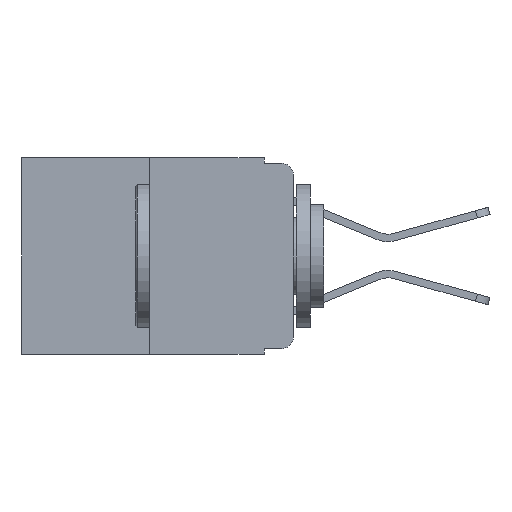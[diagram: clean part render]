
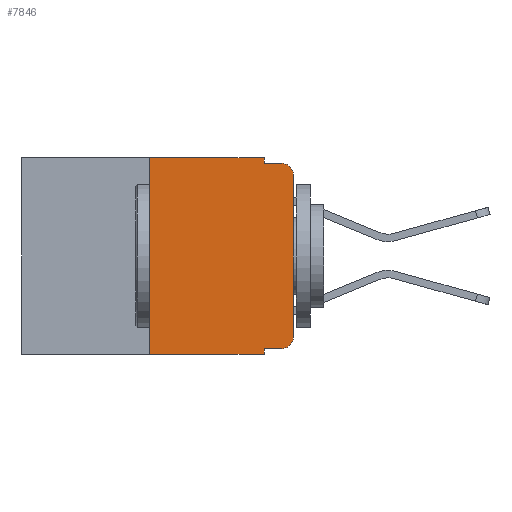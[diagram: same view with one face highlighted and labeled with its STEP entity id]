
A CAD part, left-side view. The second image highlights one B-rep face of the part: STEP entity #7846.
In plain terms, the highlighted planar face has unit normal (-1, 0, 0).
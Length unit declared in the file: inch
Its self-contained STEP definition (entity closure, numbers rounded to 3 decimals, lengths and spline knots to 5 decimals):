
#22 = ORIENTED_EDGE ( 'NONE', *, *, #587, .T. ) ;
#148 = CARTESIAN_POINT ( 'NONE',  ( 0., 0.02, -0.333 ) ) ;
#345 = CARTESIAN_POINT ( 'NONE',  ( 0., 0.25, 0. ) ) ;
#436 = LINE ( 'NONE', #345, #4178 ) ;
#462 = DIRECTION ( 'NONE',  ( -1., 0., 0. ) ) ;
#587 = EDGE_CURVE ( 'NONE', #19913, #2036, #15983, .T. ) ;
#961 = EDGE_CURVE ( 'NONE', #10880, #2807, #436, .T. ) ;
#1341 = LINE ( 'NONE', #11809, #1649 ) ;
#1512 = CARTESIAN_POINT ( 'NONE',  ( 0., 0.051, 0. ) ) ;
#1516 = CIRCLE ( 'NONE', #15545, 0.02 ) ;
#1649 = VECTOR ( 'NONE', #7474, 39.37008 ) ;
#1730 = CARTESIAN_POINT ( 'NONE',  ( 0., 0.02, -0.01 ) ) ;
#1828 = ORIENTED_EDGE ( 'NONE', *, *, #11860, .T. ) ;
#1880 = DIRECTION ( 'NONE',  ( 0., 0., 1. ) ) ;
#1892 = CARTESIAN_POINT ( 'NONE',  ( 0., 0.02, -0.03 ) ) ;
#1975 = LINE ( 'NONE', #18712, #6772 ) ;
#2036 = VERTEX_POINT ( 'NONE', #1730 ) ;
#2132 = VERTEX_POINT ( 'NONE', #8581 ) ;
#2157 = CARTESIAN_POINT ( 'NONE',  ( 0., 0.051, -0.01 ) ) ;
#2598 = ORIENTED_EDGE ( 'NONE', *, *, #6476, .T. ) ;
#2807 = VERTEX_POINT ( 'NONE', #9932 ) ;
#2822 = EDGE_CURVE ( 'NONE', #7871, #2036, #17594, .T. ) ;
#3027 = PLANE ( 'NONE',  #16008 ) ;
#3113 = LINE ( 'NONE', #6373, #11331 ) ;
#3266 = AXIS2_PLACEMENT_3D ( 'NONE', #1892, #462, #6688 ) ;
#3271 = EDGE_LOOP ( 'NONE', ( #5179, #22, #14508, #5772, #10091, #6003, #5073, #6704, #1828, #2598 ) ) ;
#3673 = VERTEX_POINT ( 'NONE', #19167 ) ;
#4142 = CARTESIAN_POINT ( 'NONE',  ( 0., 0., -0.03 ) ) ;
#4178 = VECTOR ( 'NONE', #6269, 39.37008 ) ;
#4649 = DIRECTION ( 'NONE',  ( -1., 0., 0. ) ) ;
#4750 = DIRECTION ( 'NONE',  ( 0., 0., -1. ) ) ;
#4924 = DIRECTION ( 'NONE',  ( 0., -1., 0. ) ) ;
#5021 = LINE ( 'NONE', #8103, #5763 ) ;
#5073 = ORIENTED_EDGE ( 'NONE', *, *, #7095, .T. ) ;
#5179 = ORIENTED_EDGE ( 'NONE', *, *, #17575, .T. ) ;
#5531 = LINE ( 'NONE', #17984, #15050 ) ;
#5763 = VECTOR ( 'NONE', #4924, 39.37008 ) ;
#5772 = ORIENTED_EDGE ( 'NONE', *, *, #13427, .F. ) ;
#6003 = ORIENTED_EDGE ( 'NONE', *, *, #961, .F. ) ;
#6269 = DIRECTION ( 'NONE',  ( 0., 0., 1. ) ) ;
#6373 = CARTESIAN_POINT ( 'NONE',  ( 0., 0., 0. ) ) ;
#6476 = EDGE_CURVE ( 'NONE', #18745, #8433, #1516, .T. ) ;
#6688 = DIRECTION ( 'NONE',  ( 0., 0., -1. ) ) ;
#6704 = ORIENTED_EDGE ( 'NONE', *, *, #11488, .F. ) ;
#6772 = VECTOR ( 'NONE', #17188, 39.37008 ) ;
#7095 = EDGE_CURVE ( 'NONE', #10880, #13272, #5021, .T. ) ;
#7474 = DIRECTION ( 'NONE',  ( 0., 0., -1. ) ) ;
#7618 = FACE_OUTER_BOUND ( 'NONE', #3271, .T. ) ;
#7846 = ADVANCED_FACE ( 'NONE', ( #7618 ), #3027, .F. ) ;
#7871 = VERTEX_POINT ( 'NONE', #14553 ) ;
#8103 = CARTESIAN_POINT ( 'NONE',  ( 0., 0.473, -0.343 ) ) ;
#8199 = DIRECTION ( 'NONE',  ( 0., -1., 0. ) ) ;
#8236 = DIRECTION ( 'NONE',  ( 0., 0., -1. ) ) ;
#8340 = CARTESIAN_POINT ( 'NONE',  ( 0., 0.051, -0.343 ) ) ;
#8433 = VERTEX_POINT ( 'NONE', #9941 ) ;
#8581 = CARTESIAN_POINT ( 'NONE',  ( 0., 0.051, -0.333 ) ) ;
#9063 = EDGE_CURVE ( 'NONE', #2807, #3673, #5531, .T. ) ;
#9264 = CARTESIAN_POINT ( 'NONE',  ( 0., 0.473, 0. ) ) ;
#9932 = CARTESIAN_POINT ( 'NONE',  ( 0., 0.25, 0. ) ) ;
#9941 = CARTESIAN_POINT ( 'NONE',  ( 0., 0., -0.313 ) ) ;
#10091 = ORIENTED_EDGE ( 'NONE', *, *, #9063, .F. ) ;
#10880 = VERTEX_POINT ( 'NONE', #19821 ) ;
#11331 = VECTOR ( 'NONE', #1880, 39.37008 ) ;
#11488 = EDGE_CURVE ( 'NONE', #2132, #13272, #17409, .T. ) ;
#11809 = CARTESIAN_POINT ( 'NONE',  ( 0., 0.051, 0. ) ) ;
#11860 = EDGE_CURVE ( 'NONE', #2132, #18745, #1975, .T. ) ;
#13272 = VERTEX_POINT ( 'NONE', #8340 ) ;
#13427 = EDGE_CURVE ( 'NONE', #3673, #7871, #1341, .T. ) ;
#13843 = DIRECTION ( 'NONE',  ( 0., 0., -1. ) ) ;
#14508 = ORIENTED_EDGE ( 'NONE', *, *, #2822, .F. ) ;
#14553 = CARTESIAN_POINT ( 'NONE',  ( 0., 0.051, -0.01 ) ) ;
#14564 = VECTOR ( 'NONE', #8236, 39.37008 ) ;
#15050 = VECTOR ( 'NONE', #16449, 39.37008 ) ;
#15262 = VECTOR ( 'NONE', #8199, 39.37008 ) ;
#15484 = DIRECTION ( 'NONE',  ( 1., 0., 0. ) ) ;
#15545 = AXIS2_PLACEMENT_3D ( 'NONE', #16806, #4649, #13843 ) ;
#15983 = CIRCLE ( 'NONE', #3266, 0.02 ) ;
#16008 = AXIS2_PLACEMENT_3D ( 'NONE', #9264, #15484, #4750 ) ;
#16449 = DIRECTION ( 'NONE',  ( 0., -1., 0. ) ) ;
#16806 = CARTESIAN_POINT ( 'NONE',  ( 0., 0.02, -0.313 ) ) ;
#17188 = DIRECTION ( 'NONE',  ( 0., -1., 0. ) ) ;
#17409 = LINE ( 'NONE', #1512, #14564 ) ;
#17575 = EDGE_CURVE ( 'NONE', #8433, #19913, #3113, .T. ) ;
#17594 = LINE ( 'NONE', #2157, #15262 ) ;
#17984 = CARTESIAN_POINT ( 'NONE',  ( 0., 0.473, 0. ) ) ;
#18712 = CARTESIAN_POINT ( 'NONE',  ( 0., 0.051, -0.333 ) ) ;
#18745 = VERTEX_POINT ( 'NONE', #148 ) ;
#19167 = CARTESIAN_POINT ( 'NONE',  ( 0., 0.051, 0. ) ) ;
#19821 = CARTESIAN_POINT ( 'NONE',  ( 0., 0.25, -0.343 ) ) ;
#19913 = VERTEX_POINT ( 'NONE', #4142 ) ;
